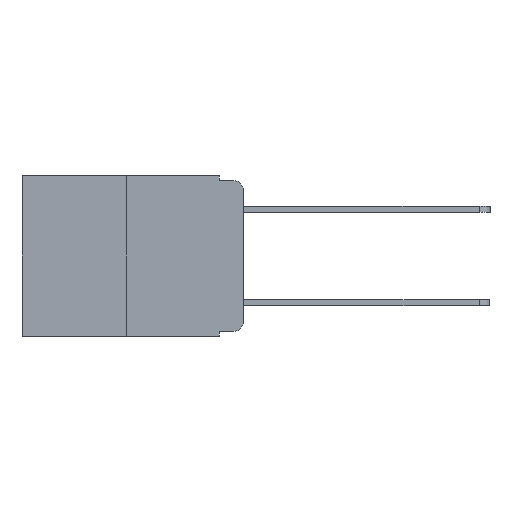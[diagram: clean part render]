
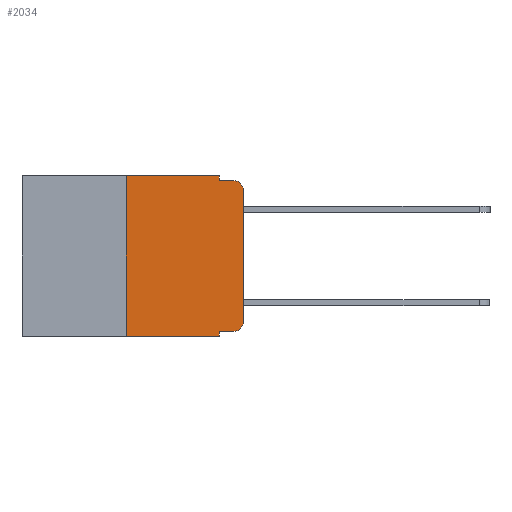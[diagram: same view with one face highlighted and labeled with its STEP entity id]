
A CAD part, left-side view. The second image highlights one B-rep face of the part: STEP entity #2034.
In plain terms, the highlighted planar face has unit normal (-1, 0, 0).
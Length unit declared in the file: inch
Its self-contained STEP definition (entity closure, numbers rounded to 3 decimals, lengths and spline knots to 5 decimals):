
#19 = EDGE_CURVE ( 'NONE', #8170, #661, #1425, .T. ) ;
#22 = EDGE_CURVE ( 'NONE', #494, #525, #6824, .T. ) ;
#47 = EDGE_CURVE ( 'NONE', #11880, #10255, #3604, .T. ) ;
#49 = EDGE_CURVE ( 'NONE', #11880, #3191, #1070, .T. ) ;
#54 = EDGE_CURVE ( 'NONE', #3191, #7880, #338, .T. ) ;
#338 = CIRCLE ( 'NONE', #7447, 0.02 ) ;
#494 = VERTEX_POINT ( 'NONE', #11777 ) ;
#525 = VERTEX_POINT ( 'NONE', #4108 ) ;
#555 = VERTEX_POINT ( 'NONE', #12062 ) ;
#661 = VERTEX_POINT ( 'NONE', #10216 ) ;
#730 = ORIENTED_EDGE ( 'NONE', *, *, #54, .T. ) ;
#736 = DIRECTION ( 'NONE',  ( 0., -1., 0. ) ) ;
#1007 = ORIENTED_EDGE ( 'NONE', *, *, #22, .F. ) ;
#1054 = CARTESIAN_POINT ( 'NONE',  ( 0., 0.02, -0.01 ) ) ;
#1070 = LINE ( 'NONE', #6070, #6279 ) ;
#1148 = CARTESIAN_POINT ( 'NONE',  ( 0., 0., -0.313 ) ) ;
#1425 = LINE ( 'NONE', #2736, #11021 ) ;
#1624 = DIRECTION ( 'NONE',  ( 0., -1., 0. ) ) ;
#2034 = ADVANCED_FACE ( 'NONE', ( #8336 ), #7903, .F. ) ;
#2039 = VECTOR ( 'NONE', #8080, 39.37008 ) ;
#2053 = CARTESIAN_POINT ( 'NONE',  ( 0., 0.473, 0. ) ) ;
#2069 = AXIS2_PLACEMENT_3D ( 'NONE', #2053, #3144, #9600 ) ;
#2148 = ORIENTED_EDGE ( 'NONE', *, *, #4187, .T. ) ;
#2541 = CIRCLE ( 'NONE', #3953, 0.02 ) ;
#2596 = ORIENTED_EDGE ( 'NONE', *, *, #49, .T. ) ;
#2672 = EDGE_CURVE ( 'NONE', #555, #6376, #2541, .T. ) ;
#2736 = CARTESIAN_POINT ( 'NONE',  ( 0., 0.051, 0. ) ) ;
#2805 = EDGE_CURVE ( 'NONE', #525, #8170, #9570, .T. ) ;
#2832 = CARTESIAN_POINT ( 'NONE',  ( 0., 0.02, -0.313 ) ) ;
#2971 = DIRECTION ( 'NONE',  ( -1., 0., 0. ) ) ;
#3032 = DIRECTION ( 'NONE',  ( -1., 0., 0. ) ) ;
#3144 = DIRECTION ( 'NONE',  ( 1., 0., 0. ) ) ;
#3178 = VECTOR ( 'NONE', #736, 39.37008 ) ;
#3191 = VERTEX_POINT ( 'NONE', #8806 ) ;
#3443 = EDGE_LOOP ( 'NONE', ( #2148, #3922, #9376, #9509, #7792, #1007, #6253, #4893, #2596, #730 ) ) ;
#3604 = LINE ( 'NONE', #10587, #10521 ) ;
#3648 = VECTOR ( 'NONE', #3970, 39.37008 ) ;
#3922 = ORIENTED_EDGE ( 'NONE', *, *, #2672, .T. ) ;
#3953 = AXIS2_PLACEMENT_3D ( 'NONE', #8667, #3032, #9520 ) ;
#3970 = DIRECTION ( 'NONE',  ( 0., 0., 1. ) ) ;
#4108 = CARTESIAN_POINT ( 'NONE',  ( 0., 0.25, 0. ) ) ;
#4187 = EDGE_CURVE ( 'NONE', #7880, #555, #6314, .T. ) ;
#4893 = ORIENTED_EDGE ( 'NONE', *, *, #47, .F. ) ;
#4974 = CARTESIAN_POINT ( 'NONE',  ( 0., 0., 0. ) ) ;
#5022 = VECTOR ( 'NONE', #1624, 39.37008 ) ;
#5335 = LINE ( 'NONE', #10899, #5022 ) ;
#5652 = CARTESIAN_POINT ( 'NONE',  ( 0., 0.051, -0.343 ) ) ;
#5906 = LINE ( 'NONE', #10248, #3178 ) ;
#6051 = EDGE_CURVE ( 'NONE', #661, #6376, #5335, .T. ) ;
#6070 = CARTESIAN_POINT ( 'NONE',  ( 0., 0.051, -0.333 ) ) ;
#6253 = ORIENTED_EDGE ( 'NONE', *, *, #9498, .T. ) ;
#6279 = VECTOR ( 'NONE', #11780, 39.37008 ) ;
#6314 = LINE ( 'NONE', #4974, #3648 ) ;
#6376 = VERTEX_POINT ( 'NONE', #1054 ) ;
#6560 = VECTOR ( 'NONE', #7390, 39.37008 ) ;
#6824 = LINE ( 'NONE', #6886, #6560 ) ;
#6886 = CARTESIAN_POINT ( 'NONE',  ( 0., 0.25, 0. ) ) ;
#7221 = CARTESIAN_POINT ( 'NONE',  ( 0., 0.473, 0. ) ) ;
#7390 = DIRECTION ( 'NONE',  ( 0., 0., 1. ) ) ;
#7447 = AXIS2_PLACEMENT_3D ( 'NONE', #2832, #2971, #9032 ) ;
#7792 = ORIENTED_EDGE ( 'NONE', *, *, #2805, .F. ) ;
#7820 = DIRECTION ( 'NONE',  ( 0., 0., -1. ) ) ;
#7880 = VERTEX_POINT ( 'NONE', #1148 ) ;
#7903 = PLANE ( 'NONE',  #2069 ) ;
#8080 = DIRECTION ( 'NONE',  ( 0., -1., 0. ) ) ;
#8170 = VERTEX_POINT ( 'NONE', #10747 ) ;
#8277 = CARTESIAN_POINT ( 'NONE',  ( 0., 0.051, -0.333 ) ) ;
#8336 = FACE_OUTER_BOUND ( 'NONE', #3443, .T. ) ;
#8667 = CARTESIAN_POINT ( 'NONE',  ( 0., 0.02, -0.03 ) ) ;
#8806 = CARTESIAN_POINT ( 'NONE',  ( 0., 0.02, -0.333 ) ) ;
#9032 = DIRECTION ( 'NONE',  ( 0., 0., -1. ) ) ;
#9376 = ORIENTED_EDGE ( 'NONE', *, *, #6051, .F. ) ;
#9498 = EDGE_CURVE ( 'NONE', #494, #10255, #5906, .T. ) ;
#9509 = ORIENTED_EDGE ( 'NONE', *, *, #19, .F. ) ;
#9520 = DIRECTION ( 'NONE',  ( 0., 0., -1. ) ) ;
#9570 = LINE ( 'NONE', #7221, #2039 ) ;
#9600 = DIRECTION ( 'NONE',  ( 0., 0., -1. ) ) ;
#10216 = CARTESIAN_POINT ( 'NONE',  ( 0., 0.051, -0.01 ) ) ;
#10248 = CARTESIAN_POINT ( 'NONE',  ( 0., 0.473, -0.343 ) ) ;
#10255 = VERTEX_POINT ( 'NONE', #5652 ) ;
#10521 = VECTOR ( 'NONE', #7820, 39.37008 ) ;
#10587 = CARTESIAN_POINT ( 'NONE',  ( 0., 0.051, 0. ) ) ;
#10747 = CARTESIAN_POINT ( 'NONE',  ( 0., 0.051, 0. ) ) ;
#10899 = CARTESIAN_POINT ( 'NONE',  ( 0., 0.051, -0.01 ) ) ;
#11021 = VECTOR ( 'NONE', #11460, 39.37008 ) ;
#11460 = DIRECTION ( 'NONE',  ( 0., 0., -1. ) ) ;
#11777 = CARTESIAN_POINT ( 'NONE',  ( 0., 0.25, -0.343 ) ) ;
#11780 = DIRECTION ( 'NONE',  ( 0., -1., 0. ) ) ;
#11880 = VERTEX_POINT ( 'NONE', #8277 ) ;
#12062 = CARTESIAN_POINT ( 'NONE',  ( 0., 0., -0.03 ) ) ;
